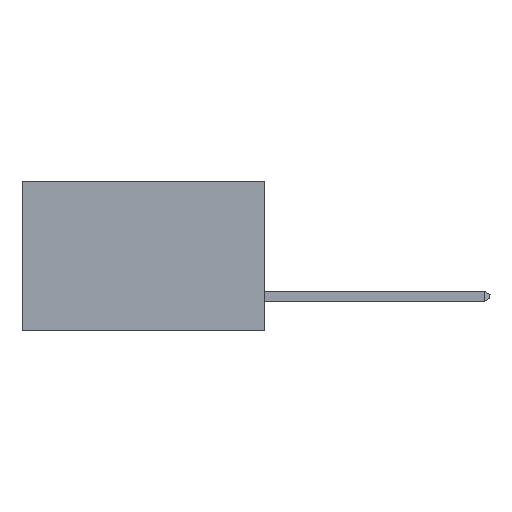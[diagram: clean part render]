
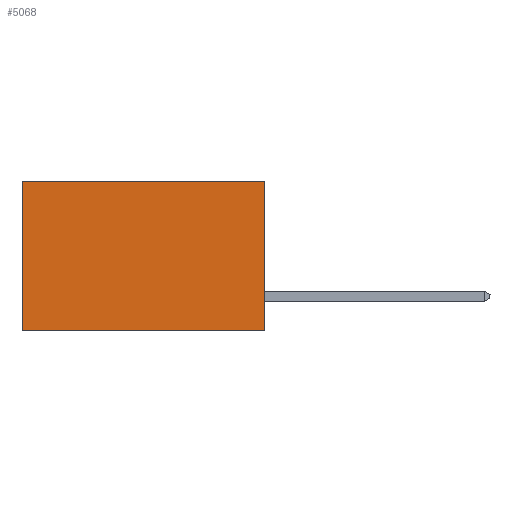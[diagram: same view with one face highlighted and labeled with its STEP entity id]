
A CAD part, left-side view. The second image highlights one B-rep face of the part: STEP entity #5068.
In plain terms, the highlighted planar face has unit normal (-1, 0, 0).
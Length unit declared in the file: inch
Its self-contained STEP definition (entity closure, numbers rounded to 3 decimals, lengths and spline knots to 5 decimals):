
#177 = VERTEX_POINT ( 'NONE', #7538 ) ;
#1264 = VECTOR ( 'NONE', #9228, 39.37008 ) ;
#1532 = LINE ( 'NONE', #8230, #13055 ) ;
#2026 = ORIENTED_EDGE ( 'NONE', *, *, #7366, .F. ) ;
#4133 = DIRECTION ( 'NONE',  ( 0., 0., -1. ) ) ;
#4375 = ORIENTED_EDGE ( 'NONE', *, *, #11235, .T. ) ;
#4551 = DIRECTION ( 'NONE',  ( 1., 0., 0. ) ) ;
#4643 = CARTESIAN_POINT ( 'NONE',  ( 0.2615, 0., -0.37 ) ) ;
#4892 = CARTESIAN_POINT ( 'NONE',  ( 0.2615, 0., -0.37 ) ) ;
#5068 = ADVANCED_FACE ( 'NONE', ( #13712 ), #11566, .F. ) ;
#5954 = DIRECTION ( 'NONE',  ( 0., 0., -1. ) ) ;
#6031 = AXIS2_PLACEMENT_3D ( 'NONE', #4643, #4551, #4133 ) ;
#6427 = EDGE_LOOP ( 'NONE', ( #9658, #14481, #2026, #4375 ) ) ;
#6788 = VECTOR ( 'NONE', #10220, 39.37008 ) ;
#6978 = DIRECTION ( 'NONE',  ( 0., 0., -1. ) ) ;
#7366 = EDGE_CURVE ( 'NONE', #7530, #177, #15546, .T. ) ;
#7530 = VERTEX_POINT ( 'NONE', #10982 ) ;
#7538 = CARTESIAN_POINT ( 'NONE',  ( 0.2615, 0., -0.37 ) ) ;
#7591 = LINE ( 'NONE', #10398, #6788 ) ;
#8113 = EDGE_CURVE ( 'NONE', #10904, #16307, #1532, .T. ) ;
#8230 = CARTESIAN_POINT ( 'NONE',  ( 0.2615, 0.6, -0.37 ) ) ;
#9187 = EDGE_CURVE ( 'NONE', #177, #16307, #7591, .T. ) ;
#9228 = DIRECTION ( 'NONE',  ( 0., 1., 0. ) ) ;
#9303 = VECTOR ( 'NONE', #5954, 39.37008 ) ;
#9658 = ORIENTED_EDGE ( 'NONE', *, *, #8113, .T. ) ;
#10220 = DIRECTION ( 'NONE',  ( 0., 1., 0. ) ) ;
#10398 = CARTESIAN_POINT ( 'NONE',  ( 0.2615, 0., -0.37 ) ) ;
#10434 = CARTESIAN_POINT ( 'NONE',  ( 0.2615, 0.6, -0.37 ) ) ;
#10672 = LINE ( 'NONE', #13099, #1264 ) ;
#10904 = VERTEX_POINT ( 'NONE', #17704 ) ;
#10982 = CARTESIAN_POINT ( 'NONE',  ( 0.2615, 0., 0. ) ) ;
#11235 = EDGE_CURVE ( 'NONE', #7530, #10904, #10672, .T. ) ;
#11566 = PLANE ( 'NONE',  #6031 ) ;
#13055 = VECTOR ( 'NONE', #6978, 39.37008 ) ;
#13099 = CARTESIAN_POINT ( 'NONE',  ( 0.2615, 0., 0. ) ) ;
#13712 = FACE_OUTER_BOUND ( 'NONE', #6427, .T. ) ;
#14481 = ORIENTED_EDGE ( 'NONE', *, *, #9187, .F. ) ;
#15546 = LINE ( 'NONE', #4892, #9303 ) ;
#16307 = VERTEX_POINT ( 'NONE', #10434 ) ;
#17704 = CARTESIAN_POINT ( 'NONE',  ( 0.2615, 0.6, 0. ) ) ;
